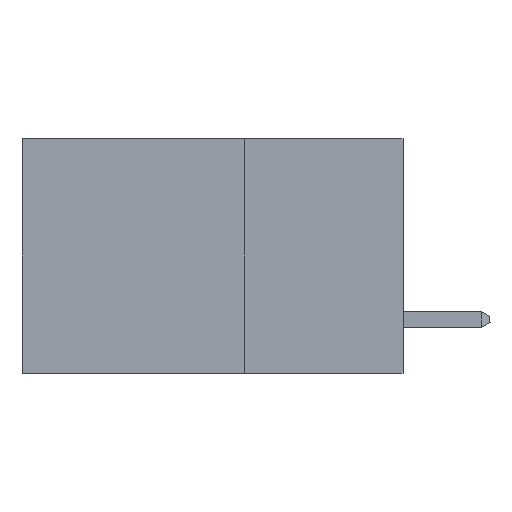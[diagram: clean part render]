
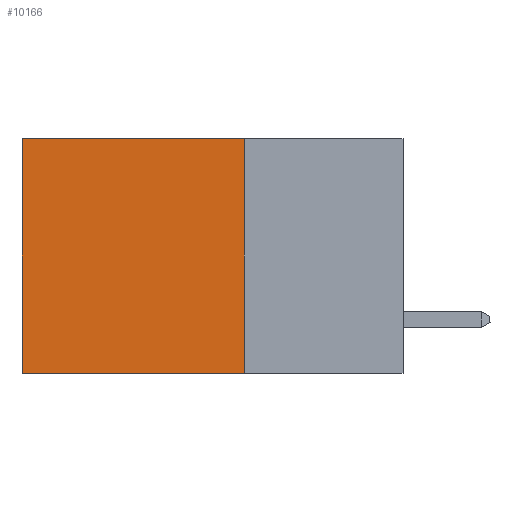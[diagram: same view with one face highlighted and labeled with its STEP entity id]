
A CAD part, left-side view. The second image highlights one B-rep face of the part: STEP entity #10166.
In plain terms, the highlighted planar face has unit normal (-1, 0, 0).
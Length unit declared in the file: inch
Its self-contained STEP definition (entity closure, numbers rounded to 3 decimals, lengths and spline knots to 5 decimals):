
#109 = EDGE_LOOP ( 'NONE', ( #5091, #19064, #14685, #10609 ) ) ;
#777 = VECTOR ( 'NONE', #7386, 39.37008 ) ;
#942 = DIRECTION ( 'NONE',  ( 0., 1., 0. ) ) ;
#1197 = CARTESIAN_POINT ( 'NONE',  ( 0.2875, 0.25, 0. ) ) ;
#1556 = CARTESIAN_POINT ( 'NONE',  ( 0.2875, 0.25, -0.37 ) ) ;
#1619 = PLANE ( 'NONE',  #18002 ) ;
#2229 = CARTESIAN_POINT ( 'NONE',  ( 0.2875, 0.6, 0. ) ) ;
#3254 = CARTESIAN_POINT ( 'NONE',  ( 0.2875, 0.6, 0. ) ) ;
#3346 = DIRECTION ( 'NONE',  ( 1., 0., 0. ) ) ;
#3614 = EDGE_CURVE ( 'NONE', #13696, #12023, #5090, .T. ) ;
#4149 = CARTESIAN_POINT ( 'NONE',  ( 0.2875, 0.25, 0. ) ) ;
#4185 = VECTOR ( 'NONE', #17397, 39.37008 ) ;
#5090 = LINE ( 'NONE', #13604, #777 ) ;
#5091 = ORIENTED_EDGE ( 'NONE', *, *, #13966, .T. ) ;
#7386 = DIRECTION ( 'NONE',  ( 0., 1., 0. ) ) ;
#7417 = LINE ( 'NONE', #2229, #11069 ) ;
#7893 = LINE ( 'NONE', #8040, #4185 ) ;
#8040 = CARTESIAN_POINT ( 'NONE',  ( 0.2875, 0.25, 0. ) ) ;
#9966 = VERTEX_POINT ( 'NONE', #1197 ) ;
#10166 = ADVANCED_FACE ( 'NONE', ( #15905 ), #1619, .F. ) ;
#10609 = ORIENTED_EDGE ( 'NONE', *, *, #16898, .T. ) ;
#11069 = VECTOR ( 'NONE', #14884, 39.37008 ) ;
#11111 = CARTESIAN_POINT ( 'NONE',  ( 0.2875, 0.6, -0.37 ) ) ;
#12023 = VERTEX_POINT ( 'NONE', #11111 ) ;
#12708 = VERTEX_POINT ( 'NONE', #3254 ) ;
#12753 = CARTESIAN_POINT ( 'NONE',  ( 0.2875, 0.25, 0. ) ) ;
#13399 = VECTOR ( 'NONE', #942, 39.37008 ) ;
#13604 = CARTESIAN_POINT ( 'NONE',  ( 0.2875, 0.25, -0.37 ) ) ;
#13696 = VERTEX_POINT ( 'NONE', #1556 ) ;
#13966 = EDGE_CURVE ( 'NONE', #12708, #12023, #7417, .T. ) ;
#14356 = DIRECTION ( 'NONE',  ( 0., 0., -1. ) ) ;
#14393 = EDGE_CURVE ( 'NONE', #9966, #13696, #7893, .T. ) ;
#14399 = LINE ( 'NONE', #4149, #13399 ) ;
#14685 = ORIENTED_EDGE ( 'NONE', *, *, #14393, .F. ) ;
#14884 = DIRECTION ( 'NONE',  ( 0., 0., -1. ) ) ;
#15905 = FACE_OUTER_BOUND ( 'NONE', #109, .T. ) ;
#16898 = EDGE_CURVE ( 'NONE', #9966, #12708, #14399, .T. ) ;
#17397 = DIRECTION ( 'NONE',  ( 0., 0., -1. ) ) ;
#18002 = AXIS2_PLACEMENT_3D ( 'NONE', #12753, #3346, #14356 ) ;
#19064 = ORIENTED_EDGE ( 'NONE', *, *, #3614, .F. ) ;
